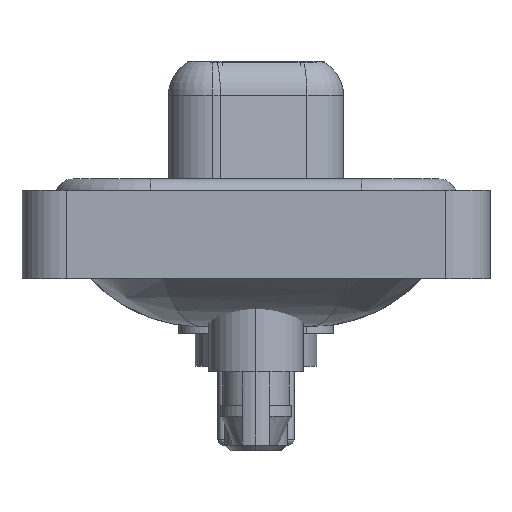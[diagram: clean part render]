
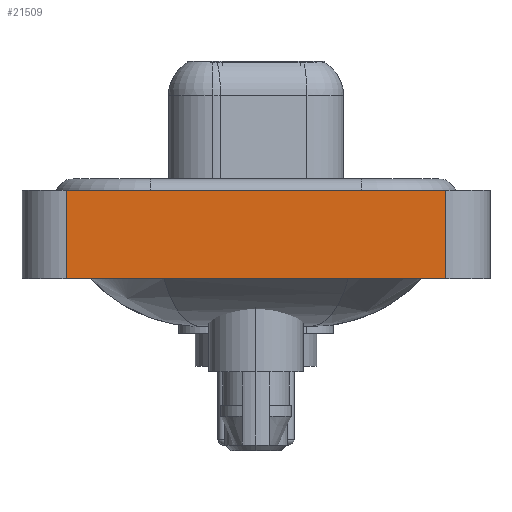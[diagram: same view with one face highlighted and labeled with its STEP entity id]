
A CAD part, left-side view. The second image highlights one B-rep face of the part: STEP entity #21509.
In plain terms, the highlighted planar face has unit normal (-1, 0, 0).
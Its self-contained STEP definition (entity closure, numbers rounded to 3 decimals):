
#936 = ORIENTED_EDGE ( 'NONE', *, *, #9365, .T. ) ;
#1049 = VERTEX_POINT ( 'NONE', #15504 ) ;
#1096 = VECTOR ( 'NONE', #1535, 1000. ) ;
#1365 = DIRECTION ( 'NONE',  ( 0., 0., 1. ) ) ;
#1535 = DIRECTION ( 'NONE',  ( 0., -1., 0. ) ) ;
#2073 = CARTESIAN_POINT ( 'NONE',  ( -7.3, 8.55, -3.6 ) ) ;
#2911 = DIRECTION ( 'NONE',  ( -1., 0., 0. ) ) ;
#2980 = CARTESIAN_POINT ( 'NONE',  ( -7.3, -8.55, -3.6 ) ) ;
#3393 = EDGE_CURVE ( 'NONE', #14434, #20327, #8580, .T. ) ;
#4123 = ORIENTED_EDGE ( 'NONE', *, *, #3393, .T. ) ;
#5057 = CARTESIAN_POINT ( 'NONE',  ( -7.3, -8.55, 0.4 ) ) ;
#5369 = LINE ( 'NONE', #5977, #14569 ) ;
#5835 = EDGE_CURVE ( 'NONE', #16957, #20327, #16113, .T. ) ;
#5977 = CARTESIAN_POINT ( 'NONE',  ( -7.3, -8.55, -3.6 ) ) ;
#7061 = DIRECTION ( 'NONE',  ( 0., 0., 1. ) ) ;
#8580 = LINE ( 'NONE', #20471, #20144 ) ;
#9365 = EDGE_CURVE ( 'NONE', #1049, #14434, #5369, .T. ) ;
#10781 = AXIS2_PLACEMENT_3D ( 'NONE', #16128, #2911, #11018 ) ;
#10978 = CARTESIAN_POINT ( 'NONE',  ( -7.3, 8.55, 0.4 ) ) ;
#11018 = DIRECTION ( 'NONE',  ( 0., 0., 1. ) ) ;
#12147 = DIRECTION ( 'NONE',  ( 0., -1., 0. ) ) ;
#14434 = VERTEX_POINT ( 'NONE', #2980 ) ;
#14569 = VECTOR ( 'NONE', #12147, 1000. ) ;
#14573 = FACE_OUTER_BOUND ( 'NONE', #18840, .T. ) ;
#15504 = CARTESIAN_POINT ( 'NONE',  ( -7.3, 8.55, -3.6 ) ) ;
#16113 = LINE ( 'NONE', #19552, #1096 ) ;
#16128 = CARTESIAN_POINT ( 'NONE',  ( -7.3, -8.55, -3.6 ) ) ;
#16232 = PLANE ( 'NONE',  #10781 ) ;
#16957 = VERTEX_POINT ( 'NONE', #10978 ) ;
#16987 = ORIENTED_EDGE ( 'NONE', *, *, #17608, .F. ) ;
#17608 = EDGE_CURVE ( 'NONE', #1049, #16957, #17654, .T. ) ;
#17654 = LINE ( 'NONE', #2073, #18128 ) ;
#18128 = VECTOR ( 'NONE', #7061, 1000. ) ;
#18840 = EDGE_LOOP ( 'NONE', ( #4123, #19444, #16987, #936 ) ) ;
#19444 = ORIENTED_EDGE ( 'NONE', *, *, #5835, .F. ) ;
#19552 = CARTESIAN_POINT ( 'NONE',  ( -7.3, -8.55, 0.4 ) ) ;
#20144 = VECTOR ( 'NONE', #1365, 1000. ) ;
#20327 = VERTEX_POINT ( 'NONE', #5057 ) ;
#20471 = CARTESIAN_POINT ( 'NONE',  ( -7.3, -8.55, -3.6 ) ) ;
#21509 = ADVANCED_FACE ( 'NONE', ( #14573 ), #16232, .T. ) ;
